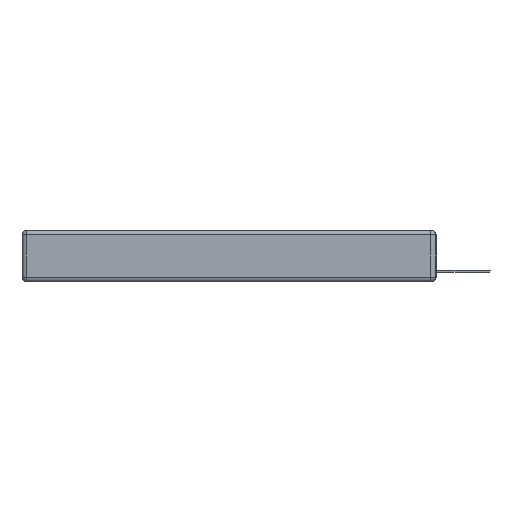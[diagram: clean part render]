
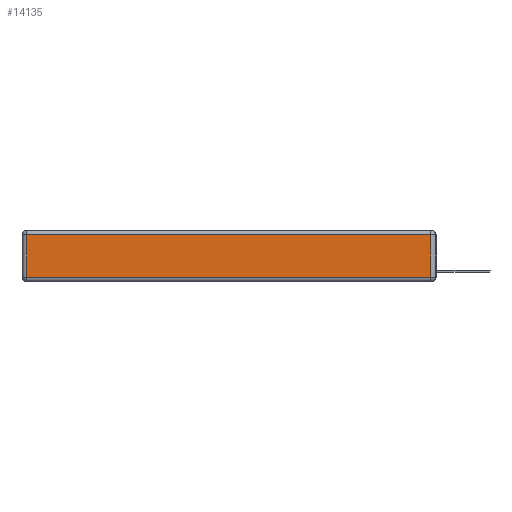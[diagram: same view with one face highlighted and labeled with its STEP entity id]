
A CAD part, left-side view. The second image highlights one B-rep face of the part: STEP entity #14135.
In plain terms, the highlighted planar face has unit normal (-1, 0, 0).
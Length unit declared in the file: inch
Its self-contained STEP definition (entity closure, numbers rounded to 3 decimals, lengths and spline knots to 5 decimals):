
#431 = VECTOR ( 'NONE', #859, 39.37008 ) ;
#525 = VERTEX_POINT ( 'NONE', #9418 ) ;
#571 = ORIENTED_EDGE ( 'NONE', *, *, #5771, .T. ) ;
#788 = VECTOR ( 'NONE', #3036, 39.37008 ) ;
#859 = DIRECTION ( 'NONE',  ( 0., 1., 0. ) ) ;
#991 = CARTESIAN_POINT ( 'NONE',  ( 0., 0., -0.343 ) ) ;
#1867 = VECTOR ( 'NONE', #2204, 39.37008 ) ;
#1910 = VERTEX_POINT ( 'NONE', #6588 ) ;
#2204 = DIRECTION ( 'NONE',  ( 0., -1., 0. ) ) ;
#3036 = DIRECTION ( 'NONE',  ( 0., 0., -1. ) ) ;
#3341 = CARTESIAN_POINT ( 'NONE',  ( 0., 0.03, -0.03 ) ) ;
#4408 = CARTESIAN_POINT ( 'NONE',  ( 0., 0.03, -0.343 ) ) ;
#4533 = DIRECTION ( 'NONE',  ( 0., 0., 1. ) ) ;
#5771 = EDGE_CURVE ( 'NONE', #8246, #7399, #15043, .T. ) ;
#6139 = FACE_OUTER_BOUND ( 'NONE', #11700, .T. ) ;
#6220 = ORIENTED_EDGE ( 'NONE', *, *, #9252, .T. ) ;
#6588 = CARTESIAN_POINT ( 'NONE',  ( 0., 2.72, -0.313 ) ) ;
#6680 = LINE ( 'NONE', #15127, #1867 ) ;
#7057 = LINE ( 'NONE', #12306, #788 ) ;
#7351 = CARTESIAN_POINT ( 'NONE',  ( 0., 0.03, -0.313 ) ) ;
#7399 = VERTEX_POINT ( 'NONE', #3341 ) ;
#7994 = LINE ( 'NONE', #13650, #431 ) ;
#8040 = PLANE ( 'NONE',  #12335 ) ;
#8246 = VERTEX_POINT ( 'NONE', #7351 ) ;
#9229 = DIRECTION ( 'NONE',  ( 0., 0., 1. ) ) ;
#9243 = DIRECTION ( 'NONE',  ( -1., 0., 0. ) ) ;
#9252 = EDGE_CURVE ( 'NONE', #7399, #525, #7994, .T. ) ;
#9418 = CARTESIAN_POINT ( 'NONE',  ( 0., 2.72, -0.03 ) ) ;
#11700 = EDGE_LOOP ( 'NONE', ( #15121, #571, #6220, #13711 ) ) ;
#12306 = CARTESIAN_POINT ( 'NONE',  ( 0., 2.72, -0.343 ) ) ;
#12335 = AXIS2_PLACEMENT_3D ( 'NONE', #991, #9243, #4533 ) ;
#13650 = CARTESIAN_POINT ( 'NONE',  ( 0., 2.75, -0.03 ) ) ;
#13711 = ORIENTED_EDGE ( 'NONE', *, *, #14482, .T. ) ;
#14135 = ADVANCED_FACE ( 'NONE', ( #6139 ), #8040, .T. ) ;
#14482 = EDGE_CURVE ( 'NONE', #525, #1910, #7057, .T. ) ;
#14821 = EDGE_CURVE ( 'NONE', #1910, #8246, #6680, .T. ) ;
#15043 = LINE ( 'NONE', #4408, #15223 ) ;
#15121 = ORIENTED_EDGE ( 'NONE', *, *, #14821, .T. ) ;
#15127 = CARTESIAN_POINT ( 'NONE',  ( 0., 0., -0.313 ) ) ;
#15223 = VECTOR ( 'NONE', #9229, 39.37008 ) ;
